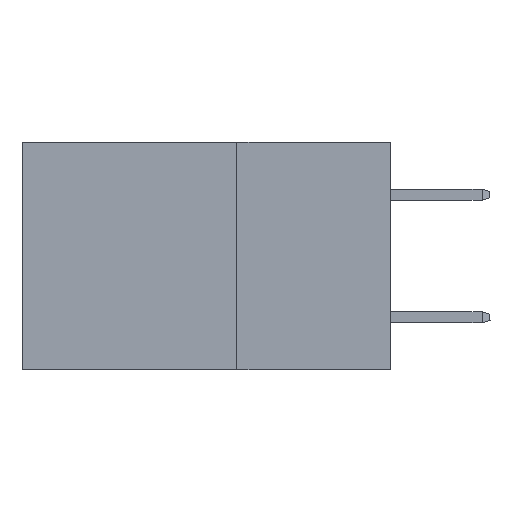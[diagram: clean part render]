
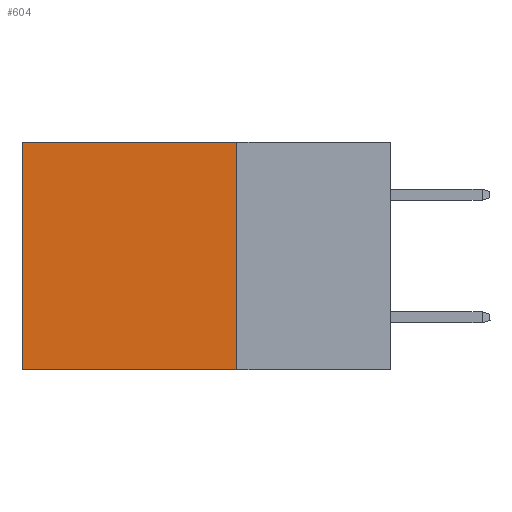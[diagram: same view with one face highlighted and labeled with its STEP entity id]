
A CAD part, left-side view. The second image highlights one B-rep face of the part: STEP entity #604.
In plain terms, the highlighted planar face has unit normal (-1, 0, 0).
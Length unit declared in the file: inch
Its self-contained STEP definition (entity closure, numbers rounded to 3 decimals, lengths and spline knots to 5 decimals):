
#604 = ADVANCED_FACE ( 'NONE', ( #3516 ), #30157, .F. ) ;
#1242 = CARTESIAN_POINT ( 'NONE',  ( 0.2875, 0.6, -0.37 ) ) ;
#2650 = CARTESIAN_POINT ( 'NONE',  ( 0.2875, 0.25, -0.37 ) ) ;
#2825 = CARTESIAN_POINT ( 'NONE',  ( 0.2875, 0.25, 0. ) ) ;
#3516 = FACE_OUTER_BOUND ( 'NONE', #19765, .T. ) ;
#3759 = DIRECTION ( 'NONE',  ( 0., 1., 0. ) ) ;
#4311 = DIRECTION ( 'NONE',  ( 0., 0., -1. ) ) ;
#4722 = EDGE_CURVE ( 'NONE', #8776, #14544, #8512, .T. ) ;
#5363 = DIRECTION ( 'NONE',  ( 0., 0., -1. ) ) ;
#5813 = CARTESIAN_POINT ( 'NONE',  ( 0.2875, 0.6, 0. ) ) ;
#8512 = LINE ( 'NONE', #26607, #14390 ) ;
#8776 = VERTEX_POINT ( 'NONE', #2650 ) ;
#11227 = CARTESIAN_POINT ( 'NONE',  ( 0.2875, 0.25, 0. ) ) ;
#11946 = CARTESIAN_POINT ( 'NONE',  ( 0.2875, 0.6, 0. ) ) ;
#12373 = ORIENTED_EDGE ( 'NONE', *, *, #20183, .T. ) ;
#13555 = ORIENTED_EDGE ( 'NONE', *, *, #4722, .F. ) ;
#14377 = DIRECTION ( 'NONE',  ( 0., 1., 0. ) ) ;
#14390 = VECTOR ( 'NONE', #14377, 39.37008 ) ;
#14544 = VERTEX_POINT ( 'NONE', #1242 ) ;
#16623 = EDGE_CURVE ( 'NONE', #18231, #22211, #26507, .T. ) ;
#18231 = VERTEX_POINT ( 'NONE', #22447 ) ;
#19765 = EDGE_LOOP ( 'NONE', ( #12373, #13555, #30987, #21623 ) ) ;
#19922 = VECTOR ( 'NONE', #3759, 39.37008 ) ;
#20183 = EDGE_CURVE ( 'NONE', #22211, #14544, #31346, .T. ) ;
#20316 = DIRECTION ( 'NONE',  ( 1., 0., 0. ) ) ;
#20644 = DIRECTION ( 'NONE',  ( 0., 0., -1. ) ) ;
#21623 = ORIENTED_EDGE ( 'NONE', *, *, #16623, .T. ) ;
#22211 = VERTEX_POINT ( 'NONE', #11946 ) ;
#22447 = CARTESIAN_POINT ( 'NONE',  ( 0.2875, 0.25, 0. ) ) ;
#24255 = CARTESIAN_POINT ( 'NONE',  ( 0.2875, 0.25, 0. ) ) ;
#26507 = LINE ( 'NONE', #11227, #19922 ) ;
#26607 = CARTESIAN_POINT ( 'NONE',  ( 0.2875, 0.25, -0.37 ) ) ;
#27980 = VECTOR ( 'NONE', #4311, 39.37008 ) ;
#29333 = AXIS2_PLACEMENT_3D ( 'NONE', #2825, #20316, #5363 ) ;
#29537 = LINE ( 'NONE', #24255, #27980 ) ;
#29639 = EDGE_CURVE ( 'NONE', #18231, #8776, #29537, .T. ) ;
#30157 = PLANE ( 'NONE',  #29333 ) ;
#30554 = VECTOR ( 'NONE', #20644, 39.37008 ) ;
#30987 = ORIENTED_EDGE ( 'NONE', *, *, #29639, .F. ) ;
#31346 = LINE ( 'NONE', #5813, #30554 ) ;
